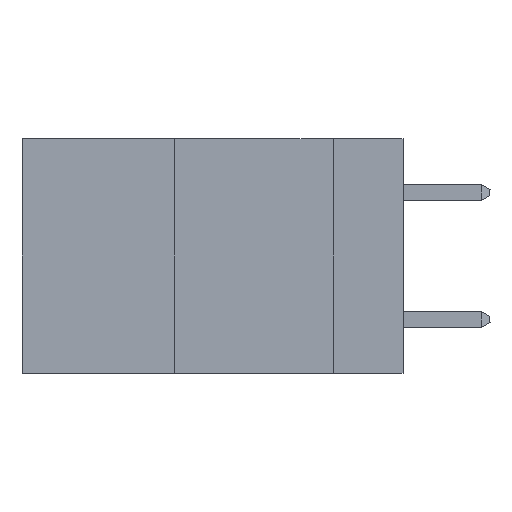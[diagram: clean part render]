
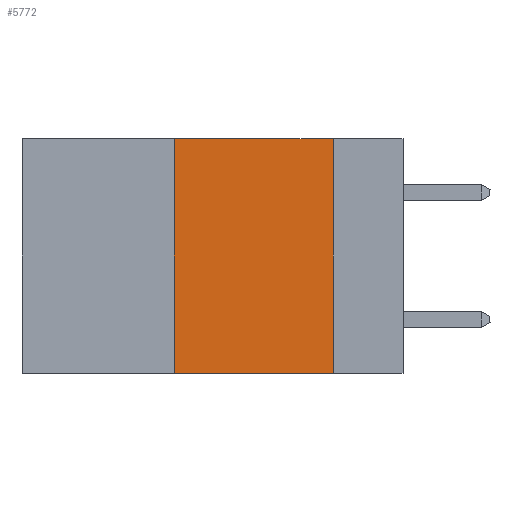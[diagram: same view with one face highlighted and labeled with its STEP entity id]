
A CAD part, left-side view. The second image highlights one B-rep face of the part: STEP entity #5772.
In plain terms, the highlighted planar face has unit normal (-1, 0, 0).
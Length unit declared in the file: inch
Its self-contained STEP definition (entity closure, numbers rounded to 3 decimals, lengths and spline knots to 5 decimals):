
#176 = VECTOR ( 'NONE', #30058, 39.37008 ) ;
#217 = EDGE_LOOP ( 'NONE', ( #29373, #19048, #36664, #10460 ) ) ;
#339 = CARTESIAN_POINT ( 'NONE',  ( 0., 0.11, 0. ) ) ;
#2451 = LINE ( 'NONE', #15517, #22806 ) ;
#5772 = ADVANCED_FACE ( 'NONE', ( #6908 ), #36256, .F. ) ;
#6908 = FACE_OUTER_BOUND ( 'NONE', #217, .T. ) ;
#7731 = CARTESIAN_POINT ( 'NONE',  ( 0., 0.36, -0.37 ) ) ;
#8783 = EDGE_CURVE ( 'NONE', #25882, #24983, #2451, .T. ) ;
#8993 = LINE ( 'NONE', #27197, #176 ) ;
#10460 = ORIENTED_EDGE ( 'NONE', *, *, #37648, .T. ) ;
#10619 = DIRECTION ( 'NONE',  ( 0., 0., -1. ) ) ;
#12871 = CARTESIAN_POINT ( 'NONE',  ( 0., 0.11, 0. ) ) ;
#13469 = CARTESIAN_POINT ( 'NONE',  ( 0., 0.6, 0. ) ) ;
#14359 = EDGE_CURVE ( 'NONE', #33464, #38106, #17934, .T. ) ;
#15517 = CARTESIAN_POINT ( 'NONE',  ( 0., 0.36, 0. ) ) ;
#16655 = VECTOR ( 'NONE', #30418, 39.37008 ) ;
#17453 = CARTESIAN_POINT ( 'NONE',  ( 0., 0.11, -0.37 ) ) ;
#17934 = LINE ( 'NONE', #339, #34606 ) ;
#19048 = ORIENTED_EDGE ( 'NONE', *, *, #29119, .F. ) ;
#21428 = DIRECTION ( 'NONE',  ( 0., 0., -1. ) ) ;
#22806 = VECTOR ( 'NONE', #30164, 39.37008 ) ;
#24983 = VERTEX_POINT ( 'NONE', #27218 ) ;
#25882 = VERTEX_POINT ( 'NONE', #7731 ) ;
#27197 = CARTESIAN_POINT ( 'NONE',  ( 0., 0.6, -0.37 ) ) ;
#27218 = CARTESIAN_POINT ( 'NONE',  ( 0., 0.36, 0. ) ) ;
#28256 = DIRECTION ( 'NONE',  ( 1., 0., 0. ) ) ;
#29119 = EDGE_CURVE ( 'NONE', #24983, #33464, #32427, .T. ) ;
#29373 = ORIENTED_EDGE ( 'NONE', *, *, #14359, .F. ) ;
#30058 = DIRECTION ( 'NONE',  ( 0., -1., 0. ) ) ;
#30164 = DIRECTION ( 'NONE',  ( 0., 0., 1. ) ) ;
#30418 = DIRECTION ( 'NONE',  ( 0., -1., 0. ) ) ;
#32427 = LINE ( 'NONE', #36080, #16655 ) ;
#33464 = VERTEX_POINT ( 'NONE', #12871 ) ;
#34606 = VECTOR ( 'NONE', #21428, 39.37008 ) ;
#34769 = AXIS2_PLACEMENT_3D ( 'NONE', #13469, #28256, #10619 ) ;
#36080 = CARTESIAN_POINT ( 'NONE',  ( 0., 0.6, 0. ) ) ;
#36256 = PLANE ( 'NONE',  #34769 ) ;
#36664 = ORIENTED_EDGE ( 'NONE', *, *, #8783, .F. ) ;
#37648 = EDGE_CURVE ( 'NONE', #25882, #38106, #8993, .T. ) ;
#38106 = VERTEX_POINT ( 'NONE', #17453 ) ;
